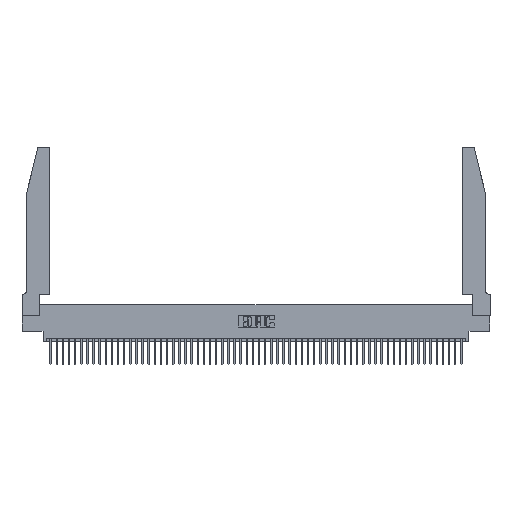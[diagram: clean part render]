
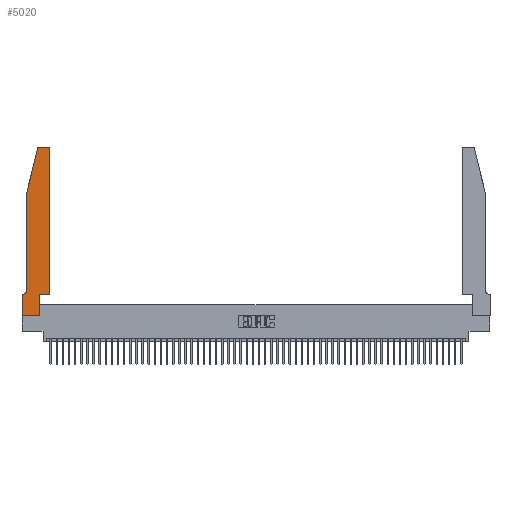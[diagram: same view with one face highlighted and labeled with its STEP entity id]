
A CAD part, top view. The second image highlights one B-rep face of the part: STEP entity #5020.
In plain terms, the highlighted planar face has unit normal (0, 0, 1).
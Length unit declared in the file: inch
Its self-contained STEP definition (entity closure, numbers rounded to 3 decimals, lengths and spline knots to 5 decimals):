
#37 = EDGE_CURVE ( 'NONE', #19106, #12249, #33434, .T. ) ;
#335 = ORIENTED_EDGE ( 'NONE', *, *, #37, .T. ) ;
#690 = EDGE_CURVE ( 'NONE', #5909, #19106, #51560, .T. ) ;
#966 = LINE ( 'NONE', #21831, #4235 ) ;
#1585 = CARTESIAN_POINT ( 'NONE',  ( 0.2605, 2.75, 0.37 ) ) ;
#2465 = DIRECTION ( 'NONE',  ( 0., 0., -1. ) ) ;
#2884 = DIRECTION ( 'NONE',  ( 0., 0., 1. ) ) ;
#3066 = PLANE ( 'NONE',  #16693 ) ;
#3093 = DIRECTION ( 'NONE',  ( 0., -1., 0. ) ) ;
#3523 = EDGE_CURVE ( 'NONE', #38377, #5909, #54671, .T. ) ;
#3604 = CARTESIAN_POINT ( 'NONE',  ( 0.284, 2.72, 0.37 ) ) ;
#3839 = CARTESIAN_POINT ( 'NONE',  ( 0.0755, 0.42, 0.37 ) ) ;
#4235 = VECTOR ( 'NONE', #43191, 39.37008 ) ;
#4918 = CIRCLE ( 'NONE', #26024, 0.03 ) ;
#5020 = ADVANCED_FACE ( 'NONE', ( #47866 ), #3066, .T. ) ;
#5205 = EDGE_CURVE ( 'NONE', #23045, #19409, #50468, .T. ) ;
#5589 = EDGE_CURVE ( 'NONE', #18437, #20235, #31847, .T. ) ;
#5721 = ORIENTED_EDGE ( 'NONE', *, *, #7042, .T. ) ;
#5909 = VERTEX_POINT ( 'NONE', #21166 ) ;
#5964 = CARTESIAN_POINT ( 'NONE',  ( 0., 0., 0.37 ) ) ;
#6040 = VERTEX_POINT ( 'NONE', #51770 ) ;
#6115 = CARTESIAN_POINT ( 'NONE',  ( 0.0055, 0.42, 0.37 ) ) ;
#6672 = CARTESIAN_POINT ( 'NONE',  ( 0.4505, 0.35, 0.37 ) ) ;
#6837 = ORIENTED_EDGE ( 'NONE', *, *, #10849, .T. ) ;
#6855 = DIRECTION ( 'NONE',  ( -1., 0., 0. ) ) ;
#7042 = EDGE_CURVE ( 'NONE', #42077, #38377, #18825, .T. ) ;
#8176 = EDGE_CURVE ( 'NONE', #27822, #42077, #966, .T. ) ;
#9409 = CARTESIAN_POINT ( 'NONE',  ( 0.4505, 0.35, 0.37 ) ) ;
#10683 = CARTESIAN_POINT ( 'NONE',  ( 0.0055, 0.35, 0.37 ) ) ;
#10849 = EDGE_CURVE ( 'NONE', #39733, #18437, #23038, .T. ) ;
#11361 = CARTESIAN_POINT ( 'NONE',  ( 0., 0., 0.37 ) ) ;
#12249 = VERTEX_POINT ( 'NONE', #52550 ) ;
#13947 = DIRECTION ( 'NONE',  ( 1., 0., 0. ) ) ;
#14774 = ORIENTED_EDGE ( 'NONE', *, *, #36952, .T. ) ;
#14775 = ORIENTED_EDGE ( 'NONE', *, *, #21224, .T. ) ;
#16693 = AXIS2_PLACEMENT_3D ( 'NONE', #45762, #2884, #32423 ) ;
#16740 = CARTESIAN_POINT ( 'NONE',  ( 0.4205, 2.72, 0.37 ) ) ;
#16919 = LINE ( 'NONE', #46179, #50710 ) ;
#17467 = ORIENTED_EDGE ( 'NONE', *, *, #5205, .T. ) ;
#18165 = CARTESIAN_POINT ( 'NONE',  ( 0.2865, 0.35, 0.37 ) ) ;
#18437 = VERTEX_POINT ( 'NONE', #9409 ) ;
#18513 = CARTESIAN_POINT ( 'NONE',  ( 0.4505, 0.35, 0.37 ) ) ;
#18570 = CARTESIAN_POINT ( 'NONE',  ( 0.284, 2.75, 0.37 ) ) ;
#18825 = CIRCLE ( 'NONE', #34484, 0.07 ) ;
#19106 = VERTEX_POINT ( 'NONE', #5964 ) ;
#19258 = ORIENTED_EDGE ( 'NONE', *, *, #43770, .T. ) ;
#19409 = VERTEX_POINT ( 'NONE', #20602 ) ;
#20235 = VERTEX_POINT ( 'NONE', #42995 ) ;
#20600 = ORIENTED_EDGE ( 'NONE', *, *, #5589, .T. ) ;
#20602 = CARTESIAN_POINT ( 'NONE',  ( 0.25487, 2.72718, 0.37 ) ) ;
#21166 = CARTESIAN_POINT ( 'NONE',  ( 0., 0.35, 0.37 ) ) ;
#21224 = EDGE_CURVE ( 'NONE', #20235, #6040, #4918, .T. ) ;
#21782 = VECTOR ( 'NONE', #26654, 39.37008 ) ;
#21831 = CARTESIAN_POINT ( 'NONE',  ( 0.0755, 2., 0.37 ) ) ;
#23038 = LINE ( 'NONE', #18513, #38986 ) ;
#23045 = VERTEX_POINT ( 'NONE', #18570 ) ;
#24337 = DIRECTION ( 'NONE',  ( 1., 0., 0. ) ) ;
#24612 = DIRECTION ( 'NONE',  ( 0., 0., 1. ) ) ;
#26024 = AXIS2_PLACEMENT_3D ( 'NONE', #16740, #53819, #24337 ) ;
#26654 = DIRECTION ( 'NONE',  ( -1., 0., 0. ) ) ;
#27822 = VERTEX_POINT ( 'NONE', #39962 ) ;
#28231 = EDGE_LOOP ( 'NONE', ( #14774, #17467, #46684, #47307, #5721, #48603, #47952, #335, #19258, #6837, #20600, #14775 ) ) ;
#30514 = DIRECTION ( 'NONE',  ( 1., 0., 0. ) ) ;
#31151 = DIRECTION ( 'NONE',  ( -1., 0., 0. ) ) ;
#31847 = LINE ( 'NONE', #6672, #45790 ) ;
#32423 = DIRECTION ( 'NONE',  ( 1., 0., 0. ) ) ;
#33113 = LINE ( 'NONE', #1585, #21782 ) ;
#33434 = LINE ( 'NONE', #52447, #42088 ) ;
#33439 = VECTOR ( 'NONE', #31151, 39.37008 ) ;
#34484 = AXIS2_PLACEMENT_3D ( 'NONE', #6115, #2465, #6855 ) ;
#34658 = LINE ( 'NONE', #18165, #45947 ) ;
#36952 = EDGE_CURVE ( 'NONE', #6040, #23045, #33113, .T. ) ;
#38377 = VERTEX_POINT ( 'NONE', #10683 ) ;
#38986 = VECTOR ( 'NONE', #13947, 39.37008 ) ;
#39733 = VERTEX_POINT ( 'NONE', #48156 ) ;
#39962 = CARTESIAN_POINT ( 'NONE',  ( 0.0755, 2., 0.37 ) ) ;
#42077 = VERTEX_POINT ( 'NONE', #3839 ) ;
#42088 = VECTOR ( 'NONE', #51712, 39.37008 ) ;
#42122 = DIRECTION ( 'NONE',  ( -0.239, -0.971, 0. ) ) ;
#42237 = EDGE_CURVE ( 'NONE', #19409, #27822, #16919, .T. ) ;
#42995 = CARTESIAN_POINT ( 'NONE',  ( 0.4505, 2.72, 0.37 ) ) ;
#43191 = DIRECTION ( 'NONE',  ( 0., -1., 0. ) ) ;
#43649 = VECTOR ( 'NONE', #3093, 39.37008 ) ;
#43770 = EDGE_CURVE ( 'NONE', #12249, #39733, #34658, .T. ) ;
#44523 = CARTESIAN_POINT ( 'NONE',  ( 0.0755, 0.35, 0.37 ) ) ;
#45762 = CARTESIAN_POINT ( 'NONE',  ( 0., 0.35, 0.37 ) ) ;
#45790 = VECTOR ( 'NONE', #48504, 39.37008 ) ;
#45947 = VECTOR ( 'NONE', #52115, 39.37008 ) ;
#46179 = CARTESIAN_POINT ( 'NONE',  ( 0.0755, 2., 0.37 ) ) ;
#46684 = ORIENTED_EDGE ( 'NONE', *, *, #42237, .T. ) ;
#47307 = ORIENTED_EDGE ( 'NONE', *, *, #8176, .T. ) ;
#47866 = FACE_OUTER_BOUND ( 'NONE', #28231, .T. ) ;
#47952 = ORIENTED_EDGE ( 'NONE', *, *, #690, .T. ) ;
#47984 = AXIS2_PLACEMENT_3D ( 'NONE', #3604, #24612, #30514 ) ;
#48156 = CARTESIAN_POINT ( 'NONE',  ( 0.2865, 0.35, 0.37 ) ) ;
#48504 = DIRECTION ( 'NONE',  ( 0., 1., 0. ) ) ;
#48603 = ORIENTED_EDGE ( 'NONE', *, *, #3523, .T. ) ;
#50468 = CIRCLE ( 'NONE', #47984, 0.03 ) ;
#50710 = VECTOR ( 'NONE', #42122, 39.37008 ) ;
#51560 = LINE ( 'NONE', #11361, #43649 ) ;
#51712 = DIRECTION ( 'NONE',  ( 1., 0., 0. ) ) ;
#51770 = CARTESIAN_POINT ( 'NONE',  ( 0.4205, 2.75, 0.37 ) ) ;
#52115 = DIRECTION ( 'NONE',  ( 0., 1., 0. ) ) ;
#52447 = CARTESIAN_POINT ( 'NONE',  ( 0., 0., 0.37 ) ) ;
#52550 = CARTESIAN_POINT ( 'NONE',  ( 0.2865, 0., 0.37 ) ) ;
#53819 = DIRECTION ( 'NONE',  ( 0., 0., 1. ) ) ;
#54671 = LINE ( 'NONE', #44523, #33439 ) ;
